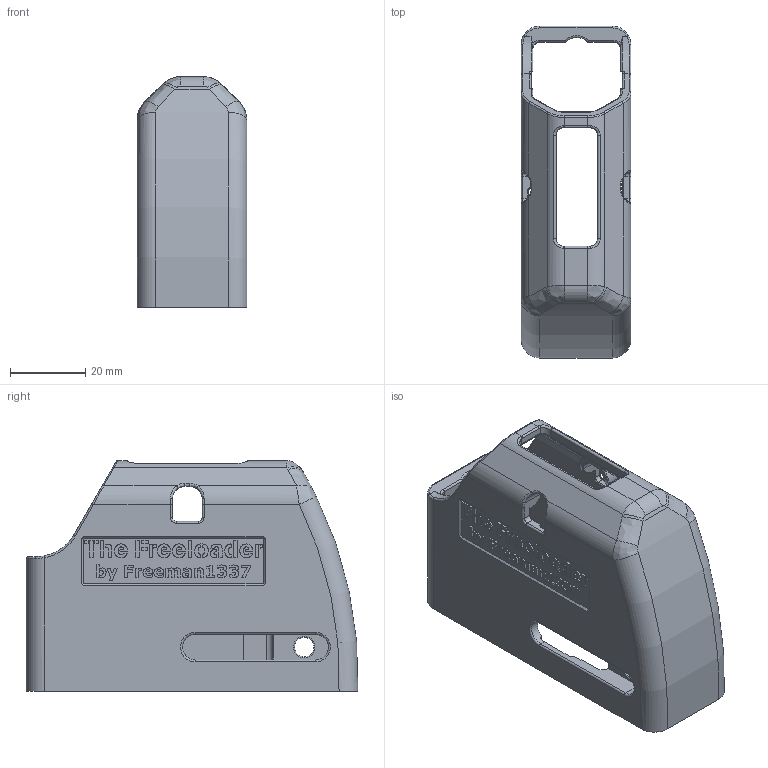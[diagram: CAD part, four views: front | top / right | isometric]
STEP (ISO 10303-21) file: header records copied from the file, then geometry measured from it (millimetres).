
FILE_DESCRIPTION(/* description */ (''),/* implementation_level */ '2;1');
FILE_NAME(/* name */ 'freeloader-body-milspec-magcatch-engraved-v3.step',/* time_stamp */ '2021-09-20T14:45:41-07:00',/* author */ (''),/* organization */ (''),/* preprocessor_version */ 'ST-DEVELOPER v18.1',/* originating_system */ 'Autodesk Translation Framework v10.10.0.1391',/* authorisation */ '');
FILE_SCHEMA (('AUTOMOTIVE_DESIGN { 1 0 10303 214 3 1 1 }'));
Products named in the file (1): loader-base-v0.3_magcatch
Bounding box: 29.22 x 88.21 x 61.31 mm (x, y, z)
Volume: 46414.7 mm3; surface area: 24524.2 mm2
Topology: 1 solids, 1 shells, 2391 faces, 6502 edges, 4277 vertices
Faces by surface type: bspline 1501, plane 706, cylinder 119, torus 59, cone 6
Full cylindrical faces by diameter (mm): 5.182 x1, 7.925 x1
Entity records: 84410 total; most frequent: CARTESIAN_POINT 35949, ORIENTED_EDGE 13004, EDGE_CURVE 6502, DIRECTION 6163, VERTEX_POINT 4277, LINE 3095, VECTOR 3095, EDGE_LOOP 2567
